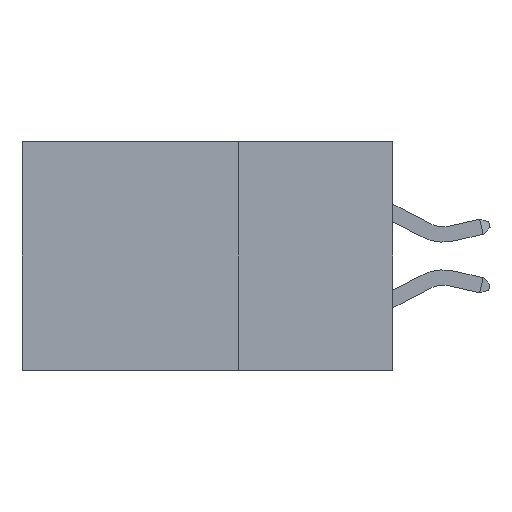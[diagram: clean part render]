
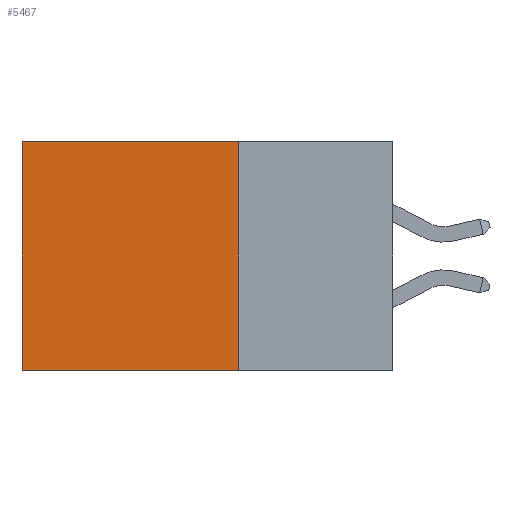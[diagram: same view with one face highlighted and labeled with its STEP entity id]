
A CAD part, left-side view. The second image highlights one B-rep face of the part: STEP entity #5467.
In plain terms, the highlighted planar face has unit normal (-1, 0, 0).
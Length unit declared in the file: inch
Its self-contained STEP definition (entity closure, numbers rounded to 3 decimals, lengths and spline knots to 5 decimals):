
#200 = EDGE_CURVE ( 'NONE', #426, #309, #8439, .T. ) ;
#309 = VERTEX_POINT ( 'NONE', #12105 ) ;
#426 = VERTEX_POINT ( 'NONE', #13493 ) ;
#718 = CARTESIAN_POINT ( 'NONE',  ( 0.2875, 0.6, 0. ) ) ;
#2458 = CARTESIAN_POINT ( 'NONE',  ( 0.2875, 0.6, 0. ) ) ;
#3334 = VECTOR ( 'NONE', #3490, 39.37008 ) ;
#3490 = DIRECTION ( 'NONE',  ( 0., 0., -1. ) ) ;
#5175 = CARTESIAN_POINT ( 'NONE',  ( 0.2875, 0.25, 0. ) ) ;
#5297 = EDGE_CURVE ( 'NONE', #7117, #5542, #9588, .T. ) ;
#5467 = ADVANCED_FACE ( 'NONE', ( #9751 ), #9817, .F. ) ;
#5517 = DIRECTION ( 'NONE',  ( 0., 0., -1. ) ) ;
#5542 = VERTEX_POINT ( 'NONE', #2458 ) ;
#6162 = DIRECTION ( 'NONE',  ( 0., 0., -1. ) ) ;
#6289 = LINE ( 'NONE', #6830, #3334 ) ;
#6830 = CARTESIAN_POINT ( 'NONE',  ( 0.2875, 0.25, 0. ) ) ;
#7117 = VERTEX_POINT ( 'NONE', #11039 ) ;
#7879 = EDGE_LOOP ( 'NONE', ( #9587, #9993, #10017, #10035 ) ) ;
#8439 = LINE ( 'NONE', #10180, #11183 ) ;
#9263 = VECTOR ( 'NONE', #13475, 39.37008 ) ;
#9345 = EDGE_CURVE ( 'NONE', #5542, #309, #11723, .T. ) ;
#9587 = ORIENTED_EDGE ( 'NONE', *, *, #9345, .T. ) ;
#9588 = LINE ( 'NONE', #5175, #9263 ) ;
#9751 = FACE_OUTER_BOUND ( 'NONE', #7879, .T. ) ;
#9817 = PLANE ( 'NONE',  #11377 ) ;
#9993 = ORIENTED_EDGE ( 'NONE', *, *, #200, .F. ) ;
#10017 = ORIENTED_EDGE ( 'NONE', *, *, #11250, .F. ) ;
#10035 = ORIENTED_EDGE ( 'NONE', *, *, #5297, .T. ) ;
#10180 = CARTESIAN_POINT ( 'NONE',  ( 0.2875, 0.25, -0.37 ) ) ;
#10243 = DIRECTION ( 'NONE',  ( 0., 1., 0. ) ) ;
#10862 = CARTESIAN_POINT ( 'NONE',  ( 0.2875, 0.25, 0. ) ) ;
#11039 = CARTESIAN_POINT ( 'NONE',  ( 0.2875, 0.25, 0. ) ) ;
#11183 = VECTOR ( 'NONE', #10243, 39.37008 ) ;
#11250 = EDGE_CURVE ( 'NONE', #7117, #426, #6289, .T. ) ;
#11377 = AXIS2_PLACEMENT_3D ( 'NONE', #10862, #11845, #5517 ) ;
#11425 = VECTOR ( 'NONE', #6162, 39.37008 ) ;
#11723 = LINE ( 'NONE', #718, #11425 ) ;
#11845 = DIRECTION ( 'NONE',  ( 1., 0., 0. ) ) ;
#12105 = CARTESIAN_POINT ( 'NONE',  ( 0.2875, 0.6, -0.37 ) ) ;
#13475 = DIRECTION ( 'NONE',  ( 0., 1., 0. ) ) ;
#13493 = CARTESIAN_POINT ( 'NONE',  ( 0.2875, 0.25, -0.37 ) ) ;
